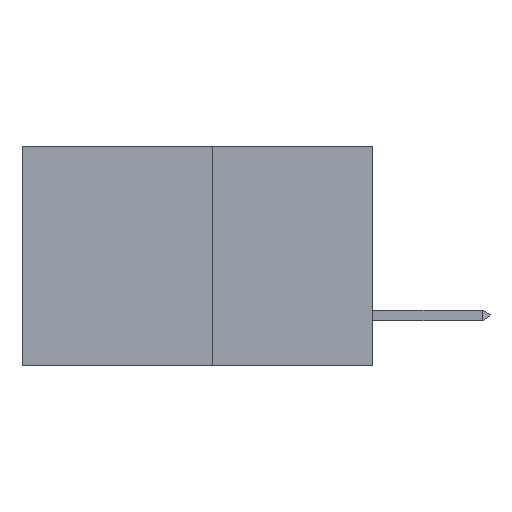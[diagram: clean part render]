
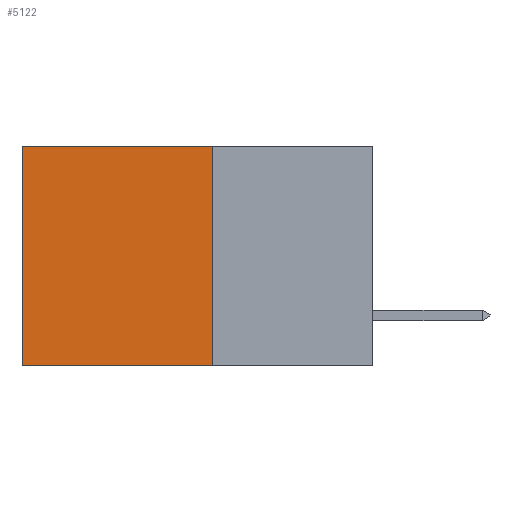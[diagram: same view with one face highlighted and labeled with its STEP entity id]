
A CAD part, left-side view. The second image highlights one B-rep face of the part: STEP entity #5122.
In plain terms, the highlighted planar face has unit normal (-1, 0, 0).
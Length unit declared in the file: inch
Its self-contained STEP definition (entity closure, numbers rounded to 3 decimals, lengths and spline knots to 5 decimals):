
#53 = FACE_OUTER_BOUND ( 'NONE', #5797, .T. ) ;
#240 = VERTEX_POINT ( 'NONE', #7962 ) ;
#471 = EDGE_CURVE ( 'NONE', #2075, #3113, #7205, .T. ) ;
#478 = VECTOR ( 'NONE', #1014, 39.37008 ) ;
#593 = CARTESIAN_POINT ( 'NONE',  ( 0.277, 0.27, 0. ) ) ;
#1014 = DIRECTION ( 'NONE',  ( 0., 1., 0. ) ) ;
#1099 = AXIS2_PLACEMENT_3D ( 'NONE', #6138, #8757, #4672 ) ;
#1269 = VERTEX_POINT ( 'NONE', #5207 ) ;
#2004 = CARTESIAN_POINT ( 'NONE',  ( 0.277, 0.59, -0.37 ) ) ;
#2075 = VERTEX_POINT ( 'NONE', #6370 ) ;
#2354 = ORIENTED_EDGE ( 'NONE', *, *, #4922, .T. ) ;
#2388 = ORIENTED_EDGE ( 'NONE', *, *, #5606, .F. ) ;
#2475 = ORIENTED_EDGE ( 'NONE', *, *, #471, .F. ) ;
#2481 = ORIENTED_EDGE ( 'NONE', *, *, #4450, .T. ) ;
#2651 = LINE ( 'NONE', #593, #478 ) ;
#3113 = VERTEX_POINT ( 'NONE', #6868 ) ;
#3902 = PLANE ( 'NONE',  #1099 ) ;
#4450 = EDGE_CURVE ( 'NONE', #2075, #1269, #2651, .T. ) ;
#4672 = DIRECTION ( 'NONE',  ( 0., 0., -1. ) ) ;
#4922 = EDGE_CURVE ( 'NONE', #1269, #240, #7431, .T. ) ;
#4999 = VECTOR ( 'NONE', #6183, 39.37008 ) ;
#5029 = DIRECTION ( 'NONE',  ( 0., 0., -1. ) ) ;
#5122 = ADVANCED_FACE ( 'NONE', ( #53 ), #3902, .F. ) ;
#5207 = CARTESIAN_POINT ( 'NONE',  ( 0.277, 0.59, 0. ) ) ;
#5417 = CARTESIAN_POINT ( 'NONE',  ( 0.277, 0.27, -0.37 ) ) ;
#5606 = EDGE_CURVE ( 'NONE', #3113, #240, #8419, .T. ) ;
#5797 = EDGE_LOOP ( 'NONE', ( #2354, #2388, #2475, #2481 ) ) ;
#5818 = DIRECTION ( 'NONE',  ( 0., 0., -1. ) ) ;
#6138 = CARTESIAN_POINT ( 'NONE',  ( 0.277, 0.27, -0.37 ) ) ;
#6183 = DIRECTION ( 'NONE',  ( 0., 1., 0. ) ) ;
#6370 = CARTESIAN_POINT ( 'NONE',  ( 0.277, 0.27, 0. ) ) ;
#6810 = VECTOR ( 'NONE', #5029, 39.37008 ) ;
#6868 = CARTESIAN_POINT ( 'NONE',  ( 0.277, 0.27, -0.37 ) ) ;
#7205 = LINE ( 'NONE', #7421, #6810 ) ;
#7421 = CARTESIAN_POINT ( 'NONE',  ( 0.277, 0.27, -0.37 ) ) ;
#7431 = LINE ( 'NONE', #2004, #9113 ) ;
#7962 = CARTESIAN_POINT ( 'NONE',  ( 0.277, 0.59, -0.37 ) ) ;
#8419 = LINE ( 'NONE', #5417, #4999 ) ;
#8757 = DIRECTION ( 'NONE',  ( 1., 0., 0. ) ) ;
#9113 = VECTOR ( 'NONE', #5818, 39.37008 ) ;
